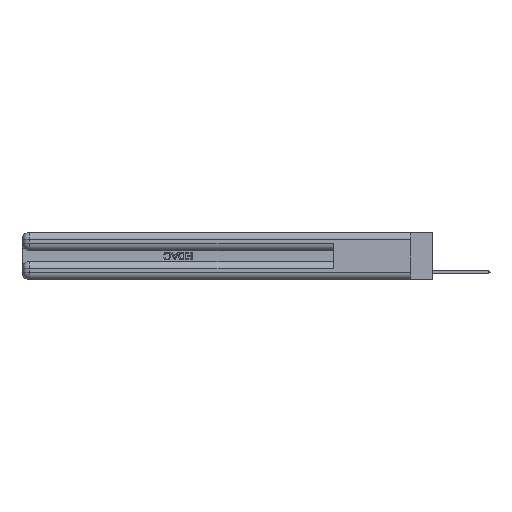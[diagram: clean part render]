
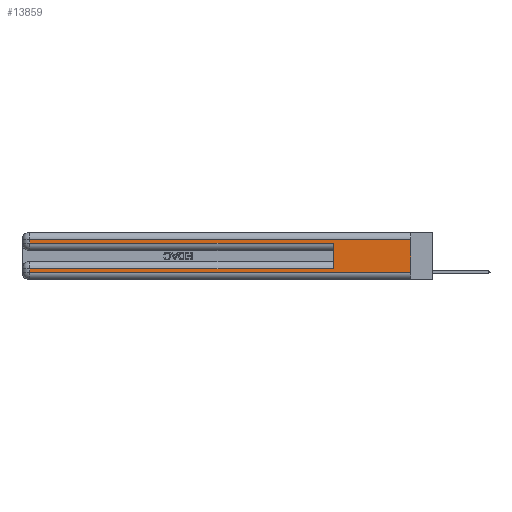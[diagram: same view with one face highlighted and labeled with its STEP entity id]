
A CAD part, left-side view. The second image highlights one B-rep face of the part: STEP entity #13859.
In plain terms, the highlighted planar face has unit normal (-1, 0, 0).
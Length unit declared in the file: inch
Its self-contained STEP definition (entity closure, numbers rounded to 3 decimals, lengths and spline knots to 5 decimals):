
#896 = CARTESIAN_POINT ( 'NONE',  ( 0., 0., 0.06 ) ) ;
#1058 = LINE ( 'NONE', #32843, #14966 ) ;
#1070 = LINE ( 'NONE', #896, #4273 ) ;
#1073 = ORIENTED_EDGE ( 'NONE', *, *, #26415, .T. ) ;
#1446 = EDGE_CURVE ( 'NONE', #24872, #6377, #7893, .T. ) ;
#1947 = CARTESIAN_POINT ( 'NONE',  ( 0., 2.94, 0.37 ) ) ;
#2262 = AXIS2_PLACEMENT_3D ( 'NONE', #23891, #16220, #3018 ) ;
#2276 = LINE ( 'NONE', #1947, #4599 ) ;
#3018 = DIRECTION ( 'NONE',  ( 0., 0., -1. ) ) ;
#3492 = ORIENTED_EDGE ( 'NONE', *, *, #6780, .T. ) ;
#4273 = VECTOR ( 'NONE', #14267, 39.37008 ) ;
#4599 = VECTOR ( 'NONE', #18034, 39.37008 ) ;
#4624 = EDGE_LOOP ( 'NONE', ( #15933, #1073, #3492, #14289, #33526, #23821, #19360, #18348 ) ) ;
#4895 = CARTESIAN_POINT ( 'NONE',  ( 0., 0.6, 0.145 ) ) ;
#5134 = EDGE_CURVE ( 'NONE', #16060, #14703, #27246, .T. ) ;
#5666 = CARTESIAN_POINT ( 'NONE',  ( 0., 0., 0.085 ) ) ;
#6377 = VERTEX_POINT ( 'NONE', #12232 ) ;
#6780 = EDGE_CURVE ( 'NONE', #26500, #16060, #12030, .T. ) ;
#7140 = EDGE_CURVE ( 'NONE', #23353, #6377, #1070, .T. ) ;
#7893 = LINE ( 'NONE', #12878, #27938 ) ;
#9469 = CARTESIAN_POINT ( 'NONE',  ( 0., 0., 0.31 ) ) ;
#9919 = CARTESIAN_POINT ( 'NONE',  ( 0., 2.94, 0.285 ) ) ;
#12030 = LINE ( 'NONE', #16982, #28039 ) ;
#12189 = CARTESIAN_POINT ( 'NONE',  ( 0., 2.94, 0.31 ) ) ;
#12232 = CARTESIAN_POINT ( 'NONE',  ( 0., 0., 0.06 ) ) ;
#12878 = CARTESIAN_POINT ( 'NONE',  ( 0., 0., 0.37 ) ) ;
#13494 = FACE_OUTER_BOUND ( 'NONE', #4624, .T. ) ;
#13859 = ADVANCED_FACE ( 'NONE', ( #13494 ), #22922, .F. ) ;
#14267 = DIRECTION ( 'NONE',  ( 0., -1., 0. ) ) ;
#14289 = ORIENTED_EDGE ( 'NONE', *, *, #5134, .T. ) ;
#14295 = CARTESIAN_POINT ( 'NONE',  ( 0., 0., 0.285 ) ) ;
#14626 = CARTESIAN_POINT ( 'NONE',  ( 0., 0.6, 0.285 ) ) ;
#14703 = VERTEX_POINT ( 'NONE', #14626 ) ;
#14966 = VECTOR ( 'NONE', #24818, 39.37008 ) ;
#15607 = DIRECTION ( 'NONE',  ( 0., 0., -1. ) ) ;
#15933 = ORIENTED_EDGE ( 'NONE', *, *, #1446, .F. ) ;
#16044 = DIRECTION ( 'NONE',  ( 0., 0., 1. ) ) ;
#16060 = VERTEX_POINT ( 'NONE', #9919 ) ;
#16220 = DIRECTION ( 'NONE',  ( 1., 0., 0. ) ) ;
#16982 = CARTESIAN_POINT ( 'NONE',  ( 0., 2.94, 0.37 ) ) ;
#18034 = DIRECTION ( 'NONE',  ( 0., 0., -1. ) ) ;
#18348 = ORIENTED_EDGE ( 'NONE', *, *, #7140, .T. ) ;
#19360 = ORIENTED_EDGE ( 'NONE', *, *, #29154, .T. ) ;
#19875 = EDGE_CURVE ( 'NONE', #25916, #14703, #31550, .T. ) ;
#19917 = DIRECTION ( 'NONE',  ( 0., -1., 0. ) ) ;
#20915 = LINE ( 'NONE', #5666, #31779 ) ;
#22438 = DIRECTION ( 'NONE',  ( 0., 0., -1. ) ) ;
#22922 = PLANE ( 'NONE',  #2262 ) ;
#23353 = VERTEX_POINT ( 'NONE', #31002 ) ;
#23821 = ORIENTED_EDGE ( 'NONE', *, *, #25144, .T. ) ;
#23891 = CARTESIAN_POINT ( 'NONE',  ( 0., 0., 0.37 ) ) ;
#24818 = DIRECTION ( 'NONE',  ( 0., 1., 0. ) ) ;
#24872 = VERTEX_POINT ( 'NONE', #9469 ) ;
#24884 = VECTOR ( 'NONE', #16044, 39.37008 ) ;
#25144 = EDGE_CURVE ( 'NONE', #25916, #30389, #20915, .T. ) ;
#25916 = VERTEX_POINT ( 'NONE', #28506 ) ;
#26194 = DIRECTION ( 'NONE',  ( 0., 1., 0. ) ) ;
#26415 = EDGE_CURVE ( 'NONE', #24872, #26500, #1058, .T. ) ;
#26500 = VERTEX_POINT ( 'NONE', #12189 ) ;
#27246 = LINE ( 'NONE', #14295, #29930 ) ;
#27938 = VECTOR ( 'NONE', #15607, 39.37008 ) ;
#28039 = VECTOR ( 'NONE', #22438, 39.37008 ) ;
#28506 = CARTESIAN_POINT ( 'NONE',  ( 0., 0.6, 0.085 ) ) ;
#29154 = EDGE_CURVE ( 'NONE', #30389, #23353, #2276, .T. ) ;
#29930 = VECTOR ( 'NONE', #19917, 39.37008 ) ;
#30389 = VERTEX_POINT ( 'NONE', #30480 ) ;
#30480 = CARTESIAN_POINT ( 'NONE',  ( 0., 2.94, 0.085 ) ) ;
#31002 = CARTESIAN_POINT ( 'NONE',  ( 0., 2.94, 0.06 ) ) ;
#31550 = LINE ( 'NONE', #4895, #24884 ) ;
#31779 = VECTOR ( 'NONE', #26194, 39.37008 ) ;
#32843 = CARTESIAN_POINT ( 'NONE',  ( 0., 0., 0.31 ) ) ;
#33526 = ORIENTED_EDGE ( 'NONE', *, *, #19875, .F. ) ;
